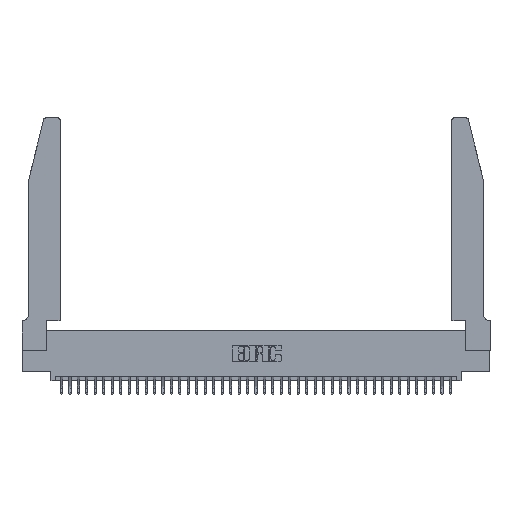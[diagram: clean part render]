
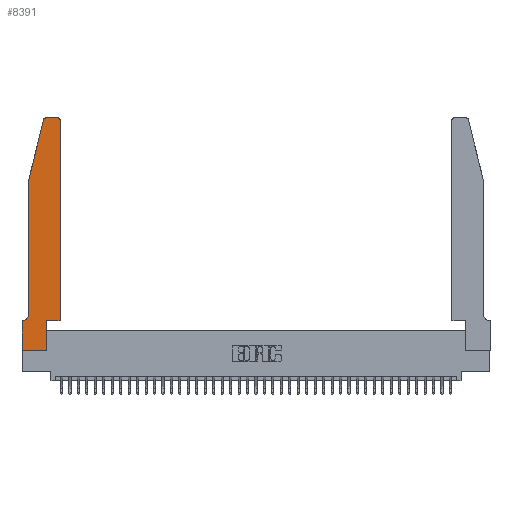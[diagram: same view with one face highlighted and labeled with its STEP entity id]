
A CAD part, top view. The second image highlights one B-rep face of the part: STEP entity #8391.
In plain terms, the highlighted planar face has unit normal (0, 0, 1).
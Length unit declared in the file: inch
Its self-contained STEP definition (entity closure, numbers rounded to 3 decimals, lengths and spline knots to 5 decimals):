
#564 = EDGE_CURVE ( 'NONE', #37537, #26704, #40544, .T. ) ;
#820 = VERTEX_POINT ( 'NONE', #9853 ) ;
#925 = EDGE_LOOP ( 'NONE', ( #30805, #3772, #18704, #6136, #3249, #19908, #12584, #22746, #27947, #5824, #38264, #28525 ) ) ;
#1110 = EDGE_CURVE ( 'NONE', #21241, #22371, #29023, .T. ) ;
#1163 = DIRECTION ( 'NONE',  ( 0., -1., 0. ) ) ;
#1851 = DIRECTION ( 'NONE',  ( 0., 1., 0. ) ) ;
#3249 = ORIENTED_EDGE ( 'NONE', *, *, #34581, .T. ) ;
#3772 = ORIENTED_EDGE ( 'NONE', *, *, #7896, .T. ) ;
#4505 = VECTOR ( 'NONE', #26457, 39.37008 ) ;
#4605 = FACE_OUTER_BOUND ( 'NONE', #925, .T. ) ;
#4888 = CARTESIAN_POINT ( 'NONE',  ( 0.0055, 0.35, 0.37 ) ) ;
#5824 = ORIENTED_EDGE ( 'NONE', *, *, #18823, .T. ) ;
#6136 = ORIENTED_EDGE ( 'NONE', *, *, #32807, .T. ) ;
#6196 = CARTESIAN_POINT ( 'NONE',  ( 0.0055, 0.42, 0.37 ) ) ;
#6326 = CARTESIAN_POINT ( 'NONE',  ( 0.4505, 0.35, 0.37 ) ) ;
#6330 = CARTESIAN_POINT ( 'NONE',  ( 0.2605, 2.75, 0.37 ) ) ;
#6748 = CARTESIAN_POINT ( 'NONE',  ( 0.284, 2.72, 0.37 ) ) ;
#7896 = EDGE_CURVE ( 'NONE', #20754, #21241, #21163, .T. ) ;
#8391 = ADVANCED_FACE ( 'NONE', ( #4605 ), #11745, .T. ) ;
#8932 = DIRECTION ( 'NONE',  ( 0., -1., 0. ) ) ;
#9017 = CARTESIAN_POINT ( 'NONE',  ( 0.0755, 2., 0.37 ) ) ;
#9705 = EDGE_CURVE ( 'NONE', #31782, #20754, #16953, .T. ) ;
#9853 = CARTESIAN_POINT ( 'NONE',  ( 0.2865, 0., 0.37 ) ) ;
#10249 = CARTESIAN_POINT ( 'NONE',  ( 0.4505, 2.72, 0.37 ) ) ;
#10651 = CARTESIAN_POINT ( 'NONE',  ( 0.0755, 0.35, 0.37 ) ) ;
#10666 = LINE ( 'NONE', #27114, #27175 ) ;
#10800 = CARTESIAN_POINT ( 'NONE',  ( 0., 0., 0.37 ) ) ;
#10898 = VECTOR ( 'NONE', #24678, 39.37008 ) ;
#11104 = AXIS2_PLACEMENT_3D ( 'NONE', #34061, #21379, #21505 ) ;
#11204 = CARTESIAN_POINT ( 'NONE',  ( 0., 0.35, 0.37 ) ) ;
#11224 = CARTESIAN_POINT ( 'NONE',  ( 0.284, 2.75, 0.37 ) ) ;
#11431 = EDGE_CURVE ( 'NONE', #820, #29256, #38396, .T. ) ;
#11745 = PLANE ( 'NONE',  #11104 ) ;
#11847 = VERTEX_POINT ( 'NONE', #23125 ) ;
#12584 = ORIENTED_EDGE ( 'NONE', *, *, #564, .T. ) ;
#12810 = LINE ( 'NONE', #34198, #13292 ) ;
#13292 = VECTOR ( 'NONE', #8932, 39.37008 ) ;
#14307 = CARTESIAN_POINT ( 'NONE',  ( 0.0755, 0.42, 0.37 ) ) ;
#14929 = VECTOR ( 'NONE', #19139, 39.37008 ) ;
#15328 = EDGE_CURVE ( 'NONE', #20118, #31782, #17637, .T. ) ;
#16712 = AXIS2_PLACEMENT_3D ( 'NONE', #6748, #35621, #38853 ) ;
#16953 = LINE ( 'NONE', #6330, #26510 ) ;
#17637 = CIRCLE ( 'NONE', #28160, 0.03 ) ;
#17980 = VECTOR ( 'NONE', #23520, 39.37008 ) ;
#18704 = ORIENTED_EDGE ( 'NONE', *, *, #1110, .T. ) ;
#18823 = EDGE_CURVE ( 'NONE', #29256, #11847, #22903, .T. ) ;
#18946 = LINE ( 'NONE', #10651, #4505 ) ;
#19139 = DIRECTION ( 'NONE',  ( 1., 0., 0. ) ) ;
#19870 = DIRECTION ( 'NONE',  ( 1., 0., 0. ) ) ;
#19908 = ORIENTED_EDGE ( 'NONE', *, *, #27041, .T. ) ;
#20105 = CARTESIAN_POINT ( 'NONE',  ( 0., 0., 0.37 ) ) ;
#20118 = VERTEX_POINT ( 'NONE', #10249 ) ;
#20593 = CARTESIAN_POINT ( 'NONE',  ( 0.0755, 2., 0.37 ) ) ;
#20754 = VERTEX_POINT ( 'NONE', #11224 ) ;
#21163 = CIRCLE ( 'NONE', #16712, 0.03 ) ;
#21241 = VERTEX_POINT ( 'NONE', #28962 ) ;
#21379 = DIRECTION ( 'NONE',  ( 0., 0., 1. ) ) ;
#21505 = DIRECTION ( 'NONE',  ( 1., 0., 0. ) ) ;
#21678 = DIRECTION ( 'NONE',  ( -1., 0., 0. ) ) ;
#22371 = VERTEX_POINT ( 'NONE', #9017 ) ;
#22732 = EDGE_CURVE ( 'NONE', #26704, #820, #37505, .T. ) ;
#22746 = ORIENTED_EDGE ( 'NONE', *, *, #22732, .T. ) ;
#22903 = LINE ( 'NONE', #6326, #14929 ) ;
#23125 = CARTESIAN_POINT ( 'NONE',  ( 0.4505, 0.35, 0.37 ) ) ;
#23520 = DIRECTION ( 'NONE',  ( 1., 0., 0. ) ) ;
#23543 = VECTOR ( 'NONE', #1163, 39.37008 ) ;
#23939 = DIRECTION ( 'NONE',  ( -0.239, -0.971, 0. ) ) ;
#24325 = AXIS2_PLACEMENT_3D ( 'NONE', #6196, #38026, #28554 ) ;
#24531 = EDGE_CURVE ( 'NONE', #11847, #20118, #10666, .T. ) ;
#24634 = CIRCLE ( 'NONE', #24325, 0.07 ) ;
#24678 = DIRECTION ( 'NONE',  ( 0., 1., 0. ) ) ;
#26457 = DIRECTION ( 'NONE',  ( -1., 0., 0. ) ) ;
#26510 = VECTOR ( 'NONE', #21678, 39.37008 ) ;
#26704 = VERTEX_POINT ( 'NONE', #34560 ) ;
#27041 = EDGE_CURVE ( 'NONE', #39978, #37537, #18946, .T. ) ;
#27092 = CARTESIAN_POINT ( 'NONE',  ( 0.2865, 0.35, 0.37 ) ) ;
#27114 = CARTESIAN_POINT ( 'NONE',  ( 0.4505, 0.35, 0.37 ) ) ;
#27175 = VECTOR ( 'NONE', #1851, 39.37008 ) ;
#27859 = CARTESIAN_POINT ( 'NONE',  ( 0.2865, 0.35, 0.37 ) ) ;
#27947 = ORIENTED_EDGE ( 'NONE', *, *, #11431, .T. ) ;
#28160 = AXIS2_PLACEMENT_3D ( 'NONE', #36211, #39430, #19870 ) ;
#28525 = ORIENTED_EDGE ( 'NONE', *, *, #15328, .T. ) ;
#28554 = DIRECTION ( 'NONE',  ( -1., 0., 0. ) ) ;
#28709 = VERTEX_POINT ( 'NONE', #14307 ) ;
#28962 = CARTESIAN_POINT ( 'NONE',  ( 0.25487, 2.72718, 0.37 ) ) ;
#29023 = LINE ( 'NONE', #20593, #32002 ) ;
#29256 = VERTEX_POINT ( 'NONE', #27859 ) ;
#30805 = ORIENTED_EDGE ( 'NONE', *, *, #9705, .T. ) ;
#31782 = VERTEX_POINT ( 'NONE', #38195 ) ;
#32002 = VECTOR ( 'NONE', #23939, 39.37008 ) ;
#32807 = EDGE_CURVE ( 'NONE', #22371, #28709, #12810, .T. ) ;
#34061 = CARTESIAN_POINT ( 'NONE',  ( 0., 0.35, 0.37 ) ) ;
#34198 = CARTESIAN_POINT ( 'NONE',  ( 0.0755, 2., 0.37 ) ) ;
#34560 = CARTESIAN_POINT ( 'NONE',  ( 0., 0., 0.37 ) ) ;
#34581 = EDGE_CURVE ( 'NONE', #28709, #39978, #24634, .T. ) ;
#35621 = DIRECTION ( 'NONE',  ( 0., 0., 1. ) ) ;
#36211 = CARTESIAN_POINT ( 'NONE',  ( 0.4205, 2.72, 0.37 ) ) ;
#37505 = LINE ( 'NONE', #10800, #17980 ) ;
#37537 = VERTEX_POINT ( 'NONE', #11204 ) ;
#38026 = DIRECTION ( 'NONE',  ( 0., 0., -1. ) ) ;
#38195 = CARTESIAN_POINT ( 'NONE',  ( 0.4205, 2.75, 0.37 ) ) ;
#38264 = ORIENTED_EDGE ( 'NONE', *, *, #24531, .T. ) ;
#38396 = LINE ( 'NONE', #27092, #10898 ) ;
#38853 = DIRECTION ( 'NONE',  ( 1., 0., 0. ) ) ;
#39430 = DIRECTION ( 'NONE',  ( 0., 0., 1. ) ) ;
#39978 = VERTEX_POINT ( 'NONE', #4888 ) ;
#40544 = LINE ( 'NONE', #20105, #23543 ) ;
